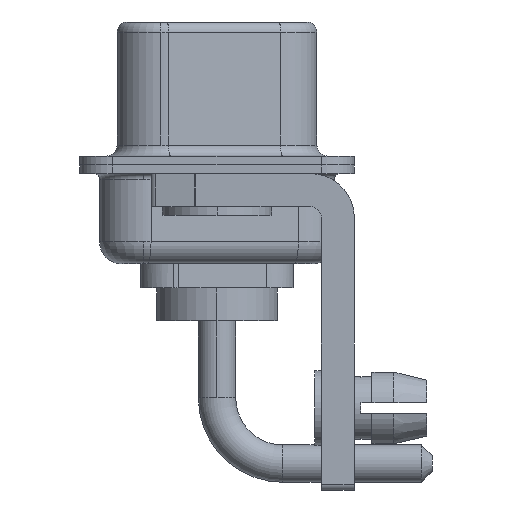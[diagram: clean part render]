
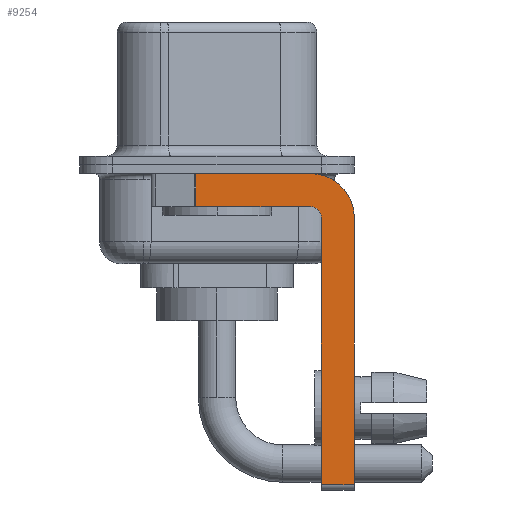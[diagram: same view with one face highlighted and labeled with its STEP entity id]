
A CAD part, left-side view. The second image highlights one B-rep face of the part: STEP entity #9254.
In plain terms, the highlighted planar face has unit normal (-1, 0, 0).
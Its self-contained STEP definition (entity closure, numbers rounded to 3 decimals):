
#248 = DIRECTION ( 'NONE',  ( 0., 0., 1. ) ) ;
#588 = EDGE_CURVE ( 'NONE', #4078, #1110, #18307, .T. ) ;
#697 = DIRECTION ( 'NONE',  ( 1., 0., 0. ) ) ;
#712 = DIRECTION ( 'NONE',  ( 0., 1., 0. ) ) ;
#1001 = VECTOR ( 'NONE', #4553, 1000. ) ;
#1110 = VERTEX_POINT ( 'NONE', #8557 ) ;
#1294 = AXIS2_PLACEMENT_3D ( 'NONE', #4155, #10345, #248 ) ;
#1298 = ORIENTED_EDGE ( 'NONE', *, *, #7741, .F. ) ;
#1887 = EDGE_CURVE ( 'NONE', #1110, #13341, #10715, .T. ) ;
#2061 = LINE ( 'NONE', #2685, #5287 ) ;
#2270 = DIRECTION ( 'NONE',  ( 0., -1., 0. ) ) ;
#2379 = CARTESIAN_POINT ( 'NONE',  ( -2.9, -4.25, -1.9 ) ) ;
#2525 = CARTESIAN_POINT ( 'NONE',  ( -2.9, -6.25, -14.55 ) ) ;
#2597 = VERTEX_POINT ( 'NONE', #4185 ) ;
#2633 = EDGE_CURVE ( 'NONE', #2694, #11082, #13168, .T. ) ;
#2685 = CARTESIAN_POINT ( 'NONE',  ( -2.9, -4.25, -14.55 ) ) ;
#2694 = VERTEX_POINT ( 'NONE', #9340 ) ;
#3009 = DIRECTION ( 'NONE',  ( 1., 0., 0. ) ) ;
#3347 = CARTESIAN_POINT ( 'NONE',  ( -2.9, -4.75, -14.55 ) ) ;
#3789 = DIRECTION ( 'NONE',  ( 0., 0., 1. ) ) ;
#4078 = VERTEX_POINT ( 'NONE', #16931 ) ;
#4155 = CARTESIAN_POINT ( 'NONE',  ( -2.9, -4.25, -2.4 ) ) ;
#4185 = CARTESIAN_POINT ( 'NONE',  ( -2.9, 0.978, -0.4 ) ) ;
#4373 = CARTESIAN_POINT ( 'NONE',  ( -2.9, -6.25, -2.4 ) ) ;
#4553 = DIRECTION ( 'NONE',  ( 0., 0., -1. ) ) ;
#4946 = LINE ( 'NONE', #16604, #10998 ) ;
#5022 = VERTEX_POINT ( 'NONE', #16422 ) ;
#5287 = VECTOR ( 'NONE', #10588, 1000. ) ;
#5881 = EDGE_CURVE ( 'NONE', #5022, #2694, #10640, .T. ) ;
#6076 = ORIENTED_EDGE ( 'NONE', *, *, #2633, .F. ) ;
#6366 = VECTOR ( 'NONE', #712, 1000. ) ;
#6555 = LINE ( 'NONE', #16473, #8281 ) ;
#6844 = ORIENTED_EDGE ( 'NONE', *, *, #7697, .T. ) ;
#7141 = VERTEX_POINT ( 'NONE', #3347 ) ;
#7446 = VECTOR ( 'NONE', #16236, 1000. ) ;
#7545 = CARTESIAN_POINT ( 'NONE',  ( -2.9, 0.978, -1.9 ) ) ;
#7697 = EDGE_CURVE ( 'NONE', #7141, #11082, #2061, .T. ) ;
#7730 = LINE ( 'NONE', #7545, #7446 ) ;
#7741 = EDGE_CURVE ( 'NONE', #7141, #4078, #4946, .T. ) ;
#8281 = VECTOR ( 'NONE', #2270, 1000. ) ;
#8557 = CARTESIAN_POINT ( 'NONE',  ( -2.9, -4.25, -1.9 ) ) ;
#8629 = EDGE_CURVE ( 'NONE', #2597, #5022, #6555, .T. ) ;
#8932 = CARTESIAN_POINT ( 'NONE',  ( -2.9, -4.25, -2.4 ) ) ;
#9254 = ADVANCED_FACE ( 'NONE', ( #17321 ), #16939, .F. ) ;
#9340 = CARTESIAN_POINT ( 'NONE',  ( -2.9, -6.25, -2.4 ) ) ;
#9414 = ORIENTED_EDGE ( 'NONE', *, *, #8629, .F. ) ;
#9960 = DIRECTION ( 'NONE',  ( 0., 0., -1. ) ) ;
#10345 = DIRECTION ( 'NONE',  ( -1., 0., 0. ) ) ;
#10542 = ORIENTED_EDGE ( 'NONE', *, *, #5881, .F. ) ;
#10588 = DIRECTION ( 'NONE',  ( 0., -1., 0. ) ) ;
#10640 = CIRCLE ( 'NONE', #13609, 2. ) ;
#10715 = LINE ( 'NONE', #2379, #6366 ) ;
#10998 = VECTOR ( 'NONE', #3789, 1000. ) ;
#11082 = VERTEX_POINT ( 'NONE', #2525 ) ;
#11805 = ORIENTED_EDGE ( 'NONE', *, *, #14799, .T. ) ;
#12105 = ORIENTED_EDGE ( 'NONE', *, *, #1887, .F. ) ;
#13168 = LINE ( 'NONE', #4373, #1001 ) ;
#13341 = VERTEX_POINT ( 'NONE', #15770 ) ;
#13609 = AXIS2_PLACEMENT_3D ( 'NONE', #8932, #697, #14891 ) ;
#14234 = CARTESIAN_POINT ( 'NONE',  ( -2.9, -4.25, -2.4 ) ) ;
#14799 = EDGE_CURVE ( 'NONE', #2597, #13341, #7730, .T. ) ;
#14891 = DIRECTION ( 'NONE',  ( 0., 0., -1. ) ) ;
#15770 = CARTESIAN_POINT ( 'NONE',  ( -2.9, 0.978, -1.9 ) ) ;
#16055 = AXIS2_PLACEMENT_3D ( 'NONE', #14234, #3009, #9960 ) ;
#16236 = DIRECTION ( 'NONE',  ( 0., 0., -1. ) ) ;
#16422 = CARTESIAN_POINT ( 'NONE',  ( -2.9, -4.25, -0.4 ) ) ;
#16473 = CARTESIAN_POINT ( 'NONE',  ( -2.9, 3., -0.4 ) ) ;
#16604 = CARTESIAN_POINT ( 'NONE',  ( -2.9, -4.75, -14.8 ) ) ;
#16931 = CARTESIAN_POINT ( 'NONE',  ( -2.9, -4.75, -2.4 ) ) ;
#16939 = PLANE ( 'NONE',  #16055 ) ;
#17166 = EDGE_LOOP ( 'NONE', ( #9414, #11805, #12105, #18124, #1298, #6844, #6076, #10542 ) ) ;
#17321 = FACE_OUTER_BOUND ( 'NONE', #17166, .T. ) ;
#18124 = ORIENTED_EDGE ( 'NONE', *, *, #588, .F. ) ;
#18307 = CIRCLE ( 'NONE', #1294, 0.5 ) ;
